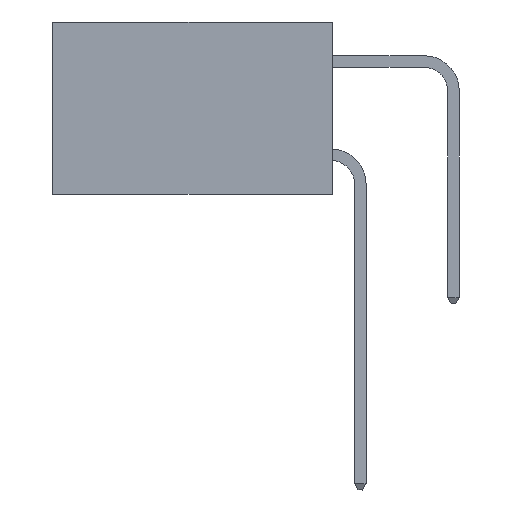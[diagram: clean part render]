
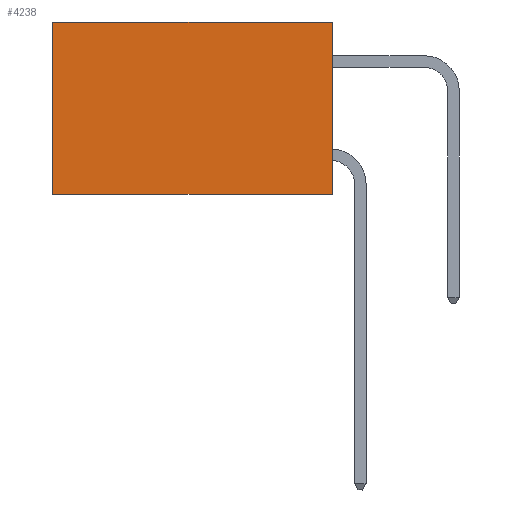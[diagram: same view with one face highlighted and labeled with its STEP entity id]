
A CAD part, left-side view. The second image highlights one B-rep face of the part: STEP entity #4238.
In plain terms, the highlighted planar face has unit normal (-1, 0, 0).
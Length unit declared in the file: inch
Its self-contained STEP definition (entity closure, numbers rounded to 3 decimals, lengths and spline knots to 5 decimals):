
#458 = CARTESIAN_POINT ( 'NONE',  ( 0.298, 0., 0. ) ) ;
#762 = LINE ( 'NONE', #10380, #17224 ) ;
#813 = LINE ( 'NONE', #18162, #23815 ) ;
#1451 = CARTESIAN_POINT ( 'NONE',  ( 0.298, 0., 0. ) ) ;
#1769 = VECTOR ( 'NONE', #14657, 39.37008 ) ;
#2271 = DIRECTION ( 'NONE',  ( 0., 0., -1. ) ) ;
#3333 = CARTESIAN_POINT ( 'NONE',  ( 0.298, 0.6, 0. ) ) ;
#4238 = ADVANCED_FACE ( 'NONE', ( #21831 ), #13815, .F. ) ;
#4847 = AXIS2_PLACEMENT_3D ( 'NONE', #458, #13583, #2271 ) ;
#7024 = LINE ( 'NONE', #1451, #10858 ) ;
#7685 = VERTEX_POINT ( 'NONE', #18452 ) ;
#8494 = VERTEX_POINT ( 'NONE', #15315 ) ;
#8813 = LINE ( 'NONE', #18320, #1769 ) ;
#9281 = CARTESIAN_POINT ( 'NONE',  ( 0.298, 0., -0.37 ) ) ;
#9867 = EDGE_LOOP ( 'NONE', ( #11302, #20654, #16317, #16328 ) ) ;
#10380 = CARTESIAN_POINT ( 'NONE',  ( 0.298, 0.6, 0. ) ) ;
#10858 = VECTOR ( 'NONE', #20107, 39.37008 ) ;
#10861 = DIRECTION ( 'NONE',  ( 0., 1., 0. ) ) ;
#11302 = ORIENTED_EDGE ( 'NONE', *, *, #16471, .T. ) ;
#11801 = EDGE_CURVE ( 'NONE', #7685, #12981, #7024, .T. ) ;
#12981 = VERTEX_POINT ( 'NONE', #9281 ) ;
#13583 = DIRECTION ( 'NONE',  ( 1., 0., 0. ) ) ;
#13815 = PLANE ( 'NONE',  #4847 ) ;
#14657 = DIRECTION ( 'NONE',  ( 0., 1., 0. ) ) ;
#15315 = CARTESIAN_POINT ( 'NONE',  ( 0.298, 0.6, -0.37 ) ) ;
#16317 = ORIENTED_EDGE ( 'NONE', *, *, #11801, .F. ) ;
#16328 = ORIENTED_EDGE ( 'NONE', *, *, #19738, .T. ) ;
#16471 = EDGE_CURVE ( 'NONE', #24360, #8494, #762, .T. ) ;
#17224 = VECTOR ( 'NONE', #19917, 39.37008 ) ;
#18162 = CARTESIAN_POINT ( 'NONE',  ( 0.298, 0., -0.37 ) ) ;
#18320 = CARTESIAN_POINT ( 'NONE',  ( 0.298, 0., 0. ) ) ;
#18452 = CARTESIAN_POINT ( 'NONE',  ( 0.298, 0., 0. ) ) ;
#19738 = EDGE_CURVE ( 'NONE', #7685, #24360, #8813, .T. ) ;
#19917 = DIRECTION ( 'NONE',  ( 0., 0., -1. ) ) ;
#20107 = DIRECTION ( 'NONE',  ( 0., 0., -1. ) ) ;
#20654 = ORIENTED_EDGE ( 'NONE', *, *, #21683, .F. ) ;
#21683 = EDGE_CURVE ( 'NONE', #12981, #8494, #813, .T. ) ;
#21831 = FACE_OUTER_BOUND ( 'NONE', #9867, .T. ) ;
#23815 = VECTOR ( 'NONE', #10861, 39.37008 ) ;
#24360 = VERTEX_POINT ( 'NONE', #3333 ) ;
